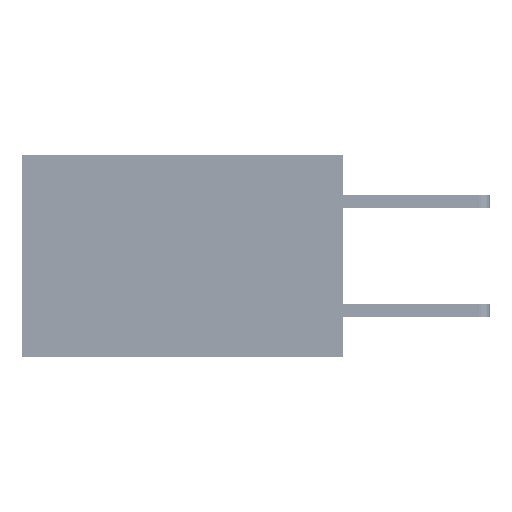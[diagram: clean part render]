
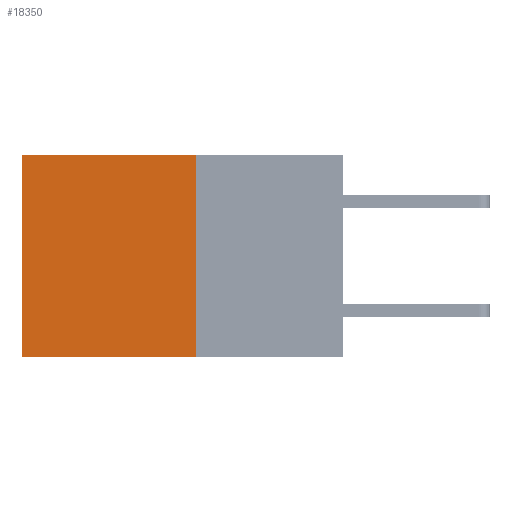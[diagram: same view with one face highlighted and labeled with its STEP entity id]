
A CAD part, left-side view. The second image highlights one B-rep face of the part: STEP entity #18350.
In plain terms, the highlighted planar face has unit normal (-1, 0, 0).
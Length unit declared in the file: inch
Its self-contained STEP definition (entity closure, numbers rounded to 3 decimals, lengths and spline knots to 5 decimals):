
#539 = CARTESIAN_POINT ( 'NONE',  ( 0.277, 0.59, 0. ) ) ;
#1155 = EDGE_CURVE ( 'NONE', #20659, #3582, #11416, .T. ) ;
#2422 = EDGE_CURVE ( 'NONE', #20659, #16133, #31262, .T. ) ;
#2805 = CARTESIAN_POINT ( 'NONE',  ( 0.277, 0.27, -0.37 ) ) ;
#3431 = VECTOR ( 'NONE', #18007, 39.37008 ) ;
#3469 = EDGE_CURVE ( 'NONE', #16133, #5244, #17963, .T. ) ;
#3582 = VERTEX_POINT ( 'NONE', #539 ) ;
#5244 = VERTEX_POINT ( 'NONE', #30903 ) ;
#5335 = ORIENTED_EDGE ( 'NONE', *, *, #2422, .F. ) ;
#6575 = DIRECTION ( 'NONE',  ( 0., 1., 0. ) ) ;
#8193 = DIRECTION ( 'NONE',  ( 1., 0., 0. ) ) ;
#9225 = AXIS2_PLACEMENT_3D ( 'NONE', #16287, #8193, #27059 ) ;
#9455 = ORIENTED_EDGE ( 'NONE', *, *, #1155, .T. ) ;
#10586 = VECTOR ( 'NONE', #34646, 39.37008 ) ;
#10726 = VECTOR ( 'NONE', #13344, 39.37008 ) ;
#11416 = LINE ( 'NONE', #22030, #27977 ) ;
#11710 = CARTESIAN_POINT ( 'NONE',  ( 0.277, 0.27, 0. ) ) ;
#13344 = DIRECTION ( 'NONE',  ( 0., 1., 0. ) ) ;
#13918 = CARTESIAN_POINT ( 'NONE',  ( 0.277, 0.27, -0.37 ) ) ;
#16133 = VERTEX_POINT ( 'NONE', #20833 ) ;
#16287 = CARTESIAN_POINT ( 'NONE',  ( 0.277, 0.27, -0.37 ) ) ;
#17963 = LINE ( 'NONE', #13918, #10726 ) ;
#18007 = DIRECTION ( 'NONE',  ( 0., 0., -1. ) ) ;
#18350 = ADVANCED_FACE ( 'NONE', ( #29024 ), #24350, .F. ) ;
#20659 = VERTEX_POINT ( 'NONE', #11710 ) ;
#20833 = CARTESIAN_POINT ( 'NONE',  ( 0.277, 0.27, -0.37 ) ) ;
#20893 = EDGE_CURVE ( 'NONE', #3582, #5244, #33032, .T. ) ;
#22030 = CARTESIAN_POINT ( 'NONE',  ( 0.277, 0.27, 0. ) ) ;
#23125 = ORIENTED_EDGE ( 'NONE', *, *, #3469, .F. ) ;
#24350 = PLANE ( 'NONE',  #9225 ) ;
#26736 = ORIENTED_EDGE ( 'NONE', *, *, #20893, .T. ) ;
#27059 = DIRECTION ( 'NONE',  ( 0., 0., -1. ) ) ;
#27977 = VECTOR ( 'NONE', #6575, 39.37008 ) ;
#29024 = FACE_OUTER_BOUND ( 'NONE', #32187, .T. ) ;
#30903 = CARTESIAN_POINT ( 'NONE',  ( 0.277, 0.59, -0.37 ) ) ;
#31262 = LINE ( 'NONE', #2805, #10586 ) ;
#31396 = CARTESIAN_POINT ( 'NONE',  ( 0.277, 0.59, -0.37 ) ) ;
#32187 = EDGE_LOOP ( 'NONE', ( #26736, #23125, #5335, #9455 ) ) ;
#33032 = LINE ( 'NONE', #31396, #3431 ) ;
#34646 = DIRECTION ( 'NONE',  ( 0., 0., -1. ) ) ;
